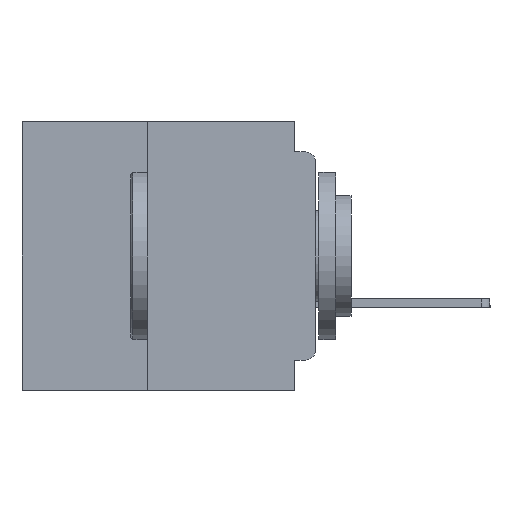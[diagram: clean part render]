
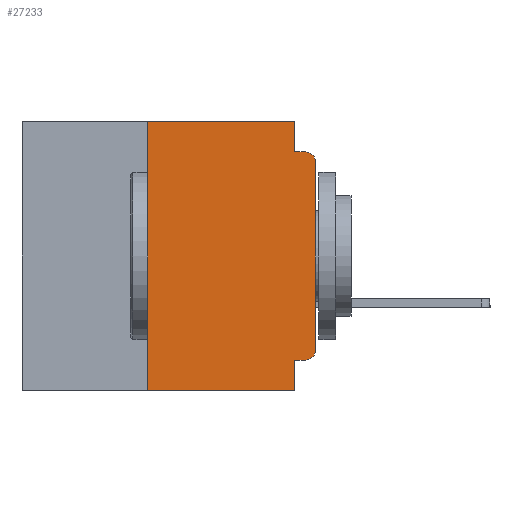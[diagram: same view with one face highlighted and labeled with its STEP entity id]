
A CAD part, left-side view. The second image highlights one B-rep face of the part: STEP entity #27233.
In plain terms, the highlighted planar face has unit normal (-1, 0, 0).
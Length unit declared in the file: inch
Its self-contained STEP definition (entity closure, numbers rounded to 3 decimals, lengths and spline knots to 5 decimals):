
#419 = EDGE_CURVE ( 'NONE', #22201, #28111, #10936, .T. ) ;
#1417 = LINE ( 'NONE', #39041, #21560 ) ;
#3413 = ORIENTED_EDGE ( 'NONE', *, *, #47126, .F. ) ;
#5427 = VERTEX_POINT ( 'NONE', #51394 ) ;
#5664 = CARTESIAN_POINT ( 'NONE',  ( 0., 0.031, -0.355 ) ) ;
#6250 = ORIENTED_EDGE ( 'NONE', *, *, #12121, .T. ) ;
#6263 = DIRECTION ( 'NONE',  ( 0., 1., 0. ) ) ;
#6616 = CARTESIAN_POINT ( 'NONE',  ( 0., 0.015, -0.06 ) ) ;
#7192 = DIRECTION ( 'NONE',  ( 0., 0., 1. ) ) ;
#9337 = DIRECTION ( 'NONE',  ( 0., -1., 0. ) ) ;
#10717 = DIRECTION ( 'NONE',  ( 0., 0., -1. ) ) ;
#10936 = LINE ( 'NONE', #39599, #28399 ) ;
#11324 = PLANE ( 'NONE',  #45603 ) ;
#12121 = EDGE_CURVE ( 'NONE', #19144, #50930, #50740, .T. ) ;
#12152 = VECTOR ( 'NONE', #6263, 39.37008 ) ;
#12474 = CARTESIAN_POINT ( 'NONE',  ( 0., 0.015, -0.34 ) ) ;
#13356 = VECTOR ( 'NONE', #17174, 39.37008 ) ;
#13715 = EDGE_CURVE ( 'NONE', #43569, #36070, #47502, .T. ) ;
#14500 = CARTESIAN_POINT ( 'NONE',  ( 0., 0.015, -0.355 ) ) ;
#14707 = VECTOR ( 'NONE', #20056, 39.37008 ) ;
#15325 = CARTESIAN_POINT ( 'NONE',  ( 0., 0.437, 0. ) ) ;
#15714 = EDGE_CURVE ( 'NONE', #22550, #5427, #26355, .T. ) ;
#16479 = DIRECTION ( 'NONE',  ( 0., 0., -1. ) ) ;
#16636 = CARTESIAN_POINT ( 'NONE',  ( 0., 0., -0.06 ) ) ;
#17174 = DIRECTION ( 'NONE',  ( 0., -1., 0. ) ) ;
#17212 = LINE ( 'NONE', #39770, #14707 ) ;
#17231 = VECTOR ( 'NONE', #49480, 39.37008 ) ;
#17706 = ORIENTED_EDGE ( 'NONE', *, *, #23699, .T. ) ;
#19144 = VERTEX_POINT ( 'NONE', #14500 ) ;
#19377 = DIRECTION ( 'NONE',  ( 0., 0., -1. ) ) ;
#19793 = CARTESIAN_POINT ( 'NONE',  ( 0., 0.031, -0.4 ) ) ;
#20056 = DIRECTION ( 'NONE',  ( 0., 0., 1. ) ) ;
#21224 = FACE_OUTER_BOUND ( 'NONE', #48190, .T. ) ;
#21560 = VECTOR ( 'NONE', #50746, 39.37008 ) ;
#22201 = VERTEX_POINT ( 'NONE', #38183 ) ;
#22325 = ORIENTED_EDGE ( 'NONE', *, *, #24213, .F. ) ;
#22443 = DIRECTION ( 'NONE',  ( 0., 0., -1. ) ) ;
#22550 = VERTEX_POINT ( 'NONE', #16636 ) ;
#22789 = LINE ( 'NONE', #42125, #12152 ) ;
#23699 = EDGE_CURVE ( 'NONE', #50930, #22550, #17212, .T. ) ;
#24213 = EDGE_CURVE ( 'NONE', #46088, #22201, #1417, .T. ) ;
#24862 = CARTESIAN_POINT ( 'NONE',  ( 0., 0.25, -0.4 ) ) ;
#24882 = VECTOR ( 'NONE', #7192, 39.37008 ) ;
#26355 = CIRCLE ( 'NONE', #47029, 0.015 ) ;
#27093 = AXIS2_PLACEMENT_3D ( 'NONE', #12474, #40259, #16479 ) ;
#27233 = ADVANCED_FACE ( 'NONE', ( #21224 ), #11324, .F. ) ;
#27407 = ORIENTED_EDGE ( 'NONE', *, *, #35835, .F. ) ;
#28026 = VECTOR ( 'NONE', #9337, 39.37008 ) ;
#28111 = VERTEX_POINT ( 'NONE', #48470 ) ;
#28399 = VECTOR ( 'NONE', #22443, 39.37008 ) ;
#29262 = CARTESIAN_POINT ( 'NONE',  ( 0., 0., -0.045 ) ) ;
#31158 = CARTESIAN_POINT ( 'NONE',  ( 0., 0.25, -0.4 ) ) ;
#32833 = ORIENTED_EDGE ( 'NONE', *, *, #419, .F. ) ;
#33003 = CARTESIAN_POINT ( 'NONE',  ( 0., 0., -0.34 ) ) ;
#33653 = CARTESIAN_POINT ( 'NONE',  ( 0., 0.031, -0.4 ) ) ;
#34550 = DIRECTION ( 'NONE',  ( -1., 0., 0. ) ) ;
#35835 = EDGE_CURVE ( 'NONE', #19144, #36857, #22789, .T. ) ;
#36070 = VERTEX_POINT ( 'NONE', #19793 ) ;
#36644 = LINE ( 'NONE', #31158, #24882 ) ;
#36857 = VERTEX_POINT ( 'NONE', #5664 ) ;
#36979 = CARTESIAN_POINT ( 'NONE',  ( 0., 0.437, -0.4 ) ) ;
#38183 = CARTESIAN_POINT ( 'NONE',  ( 0., 0.031, 0. ) ) ;
#38887 = ORIENTED_EDGE ( 'NONE', *, *, #42997, .F. ) ;
#39041 = CARTESIAN_POINT ( 'NONE',  ( 0., 0.437, 0. ) ) ;
#39555 = ORIENTED_EDGE ( 'NONE', *, *, #15714, .T. ) ;
#39599 = CARTESIAN_POINT ( 'NONE',  ( 0., 0.031, 0. ) ) ;
#39747 = LINE ( 'NONE', #29262, #28026 ) ;
#39770 = CARTESIAN_POINT ( 'NONE',  ( 0., 0., 0. ) ) ;
#40259 = DIRECTION ( 'NONE',  ( -1., 0., 0. ) ) ;
#40819 = LINE ( 'NONE', #33653, #17231 ) ;
#42125 = CARTESIAN_POINT ( 'NONE',  ( 0., 0., -0.355 ) ) ;
#42997 = EDGE_CURVE ( 'NONE', #28111, #5427, #39747, .T. ) ;
#43070 = CARTESIAN_POINT ( 'NONE',  ( 0., 0.25, 0. ) ) ;
#43094 = DIRECTION ( 'NONE',  ( 1., 0., 0. ) ) ;
#43291 = EDGE_CURVE ( 'NONE', #43569, #46088, #36644, .T. ) ;
#43569 = VERTEX_POINT ( 'NONE', #24862 ) ;
#45603 = AXIS2_PLACEMENT_3D ( 'NONE', #15325, #43094, #19377 ) ;
#46088 = VERTEX_POINT ( 'NONE', #43070 ) ;
#47029 = AXIS2_PLACEMENT_3D ( 'NONE', #6616, #34550, #10717 ) ;
#47126 = EDGE_CURVE ( 'NONE', #36857, #36070, #40819, .T. ) ;
#47337 = ORIENTED_EDGE ( 'NONE', *, *, #43291, .F. ) ;
#47502 = LINE ( 'NONE', #36979, #13356 ) ;
#48190 = EDGE_LOOP ( 'NONE', ( #17706, #39555, #38887, #32833, #22325, #47337, #48580, #3413, #27407, #6250 ) ) ;
#48470 = CARTESIAN_POINT ( 'NONE',  ( 0., 0.031, -0.045 ) ) ;
#48580 = ORIENTED_EDGE ( 'NONE', *, *, #13715, .T. ) ;
#49480 = DIRECTION ( 'NONE',  ( 0., 0., -1. ) ) ;
#50740 = CIRCLE ( 'NONE', #27093, 0.015 ) ;
#50746 = DIRECTION ( 'NONE',  ( 0., -1., 0. ) ) ;
#50930 = VERTEX_POINT ( 'NONE', #33003 ) ;
#51394 = CARTESIAN_POINT ( 'NONE',  ( 0., 0.015, -0.045 ) ) ;
